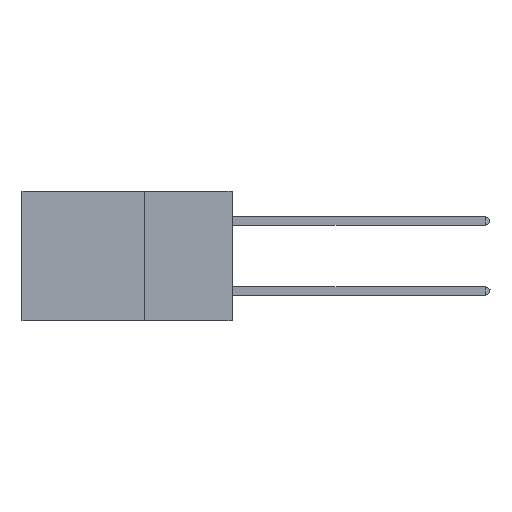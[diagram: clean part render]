
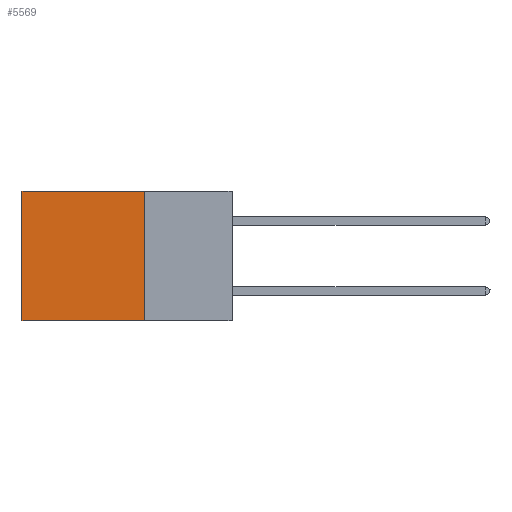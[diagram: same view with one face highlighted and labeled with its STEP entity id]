
A CAD part, left-side view. The second image highlights one B-rep face of the part: STEP entity #5569.
In plain terms, the highlighted planar face has unit normal (-1, 0, 0).
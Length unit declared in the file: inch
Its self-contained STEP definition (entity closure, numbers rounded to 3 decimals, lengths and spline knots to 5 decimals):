
#548 = ORIENTED_EDGE ( 'NONE', *, *, #7240, .F. ) ;
#1098 = ORIENTED_EDGE ( 'NONE', *, *, #12723, .T. ) ;
#1335 = VERTEX_POINT ( 'NONE', #21616 ) ;
#2900 = DIRECTION ( 'NONE',  ( 0., 1., 0. ) ) ;
#3147 = ORIENTED_EDGE ( 'NONE', *, *, #13142, .T. ) ;
#3645 = VECTOR ( 'NONE', #13359, 39.37008 ) ;
#3811 = CARTESIAN_POINT ( 'NONE',  ( 0.2875, 0.25, -0.37 ) ) ;
#4845 = DIRECTION ( 'NONE',  ( 0., 1., 0. ) ) ;
#4954 = CARTESIAN_POINT ( 'NONE',  ( 0.2875, 0.25, 0. ) ) ;
#5039 = CARTESIAN_POINT ( 'NONE',  ( 0.2875, 0.25, 0. ) ) ;
#5569 = ADVANCED_FACE ( 'NONE', ( #9733 ), #13400, .F. ) ;
#6185 = CARTESIAN_POINT ( 'NONE',  ( 0.2875, 0.25, 0. ) ) ;
#7240 = EDGE_CURVE ( 'NONE', #16598, #1335, #20797, .T. ) ;
#8020 = CARTESIAN_POINT ( 'NONE',  ( 0.2875, 0.6, 0. ) ) ;
#8352 = VERTEX_POINT ( 'NONE', #14408 ) ;
#8742 = VECTOR ( 'NONE', #4845, 39.37008 ) ;
#9190 = LINE ( 'NONE', #6185, #17319 ) ;
#9733 = FACE_OUTER_BOUND ( 'NONE', #12438, .T. ) ;
#10367 = VERTEX_POINT ( 'NONE', #4954 ) ;
#10561 = AXIS2_PLACEMENT_3D ( 'NONE', #5039, #16516, #16796 ) ;
#11535 = CARTESIAN_POINT ( 'NONE',  ( 0.2875, 0.25, 0. ) ) ;
#12438 = EDGE_LOOP ( 'NONE', ( #3147, #548, #15552, #1098 ) ) ;
#12723 = EDGE_CURVE ( 'NONE', #10367, #8352, #9190, .T. ) ;
#13078 = LINE ( 'NONE', #8020, #21488 ) ;
#13142 = EDGE_CURVE ( 'NONE', #8352, #1335, #13078, .T. ) ;
#13359 = DIRECTION ( 'NONE',  ( 0., 0., -1. ) ) ;
#13400 = PLANE ( 'NONE',  #10561 ) ;
#14408 = CARTESIAN_POINT ( 'NONE',  ( 0.2875, 0.6, 0. ) ) ;
#14921 = CARTESIAN_POINT ( 'NONE',  ( 0.2875, 0.25, -0.37 ) ) ;
#15552 = ORIENTED_EDGE ( 'NONE', *, *, #21221, .F. ) ;
#16516 = DIRECTION ( 'NONE',  ( 1., 0., 0. ) ) ;
#16598 = VERTEX_POINT ( 'NONE', #3811 ) ;
#16796 = DIRECTION ( 'NONE',  ( 0., 0., -1. ) ) ;
#17319 = VECTOR ( 'NONE', #2900, 39.37008 ) ;
#18120 = DIRECTION ( 'NONE',  ( 0., 0., -1. ) ) ;
#20215 = LINE ( 'NONE', #11535, #3645 ) ;
#20797 = LINE ( 'NONE', #14921, #8742 ) ;
#21221 = EDGE_CURVE ( 'NONE', #10367, #16598, #20215, .T. ) ;
#21488 = VECTOR ( 'NONE', #18120, 39.37008 ) ;
#21616 = CARTESIAN_POINT ( 'NONE',  ( 0.2875, 0.6, -0.37 ) ) ;
